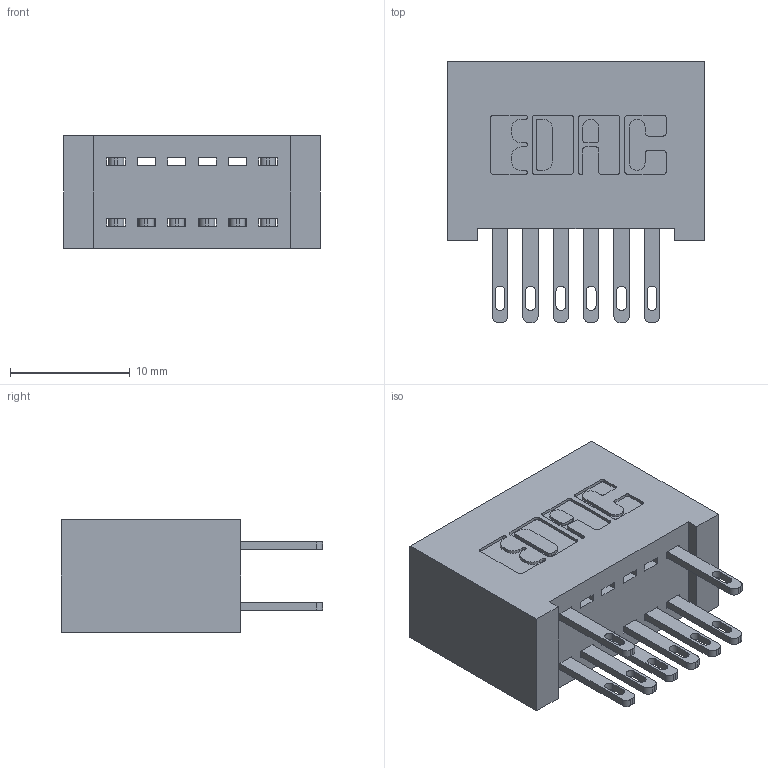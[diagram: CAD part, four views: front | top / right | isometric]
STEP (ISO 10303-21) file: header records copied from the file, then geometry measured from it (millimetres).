
FILE_DESCRIPTION (( 'STEP AP203' ), '1' );
FILE_NAME ('342-012-500-201.STEP', '2018-08-10T14:48:07', ( '' ), ( '' ), 'SwSTEP 2.0', 'SolidWorks 2016', '' );
FILE_SCHEMA (( 'CONFIG_CONTROL_DESIGN' ));
Length unit declared in the file: inch
Products named in the file (3): 342 Part_Lugless; 345-292-001_345-293-100; 342-012-500-201
Assembly tree (9 placements, depth 2):
  342-012-500-201
    342 Part_Lugless
    345-292-001_345-293-100  x8
Bounding box: 21.49 x 21.85 x 9.4 mm (x, y, z)
Volume: 2188.3 mm3; surface area: 2998.8 mm2
Topology: 9 solids, 9 shells, 510 faces, 1535 edges, 1022 vertices
Faces by surface type: plane 326, cylinder 184
Entity records: 7909 total; most frequent: CARTESIAN_POINT 1366, ORIENTED_EDGE 1306, DIRECTION 1221, EDGE_CURVE 653, VECTOR 529, LINE 529, VERTEX_POINT 434, AXIS2_PLACEMENT_3D 346
